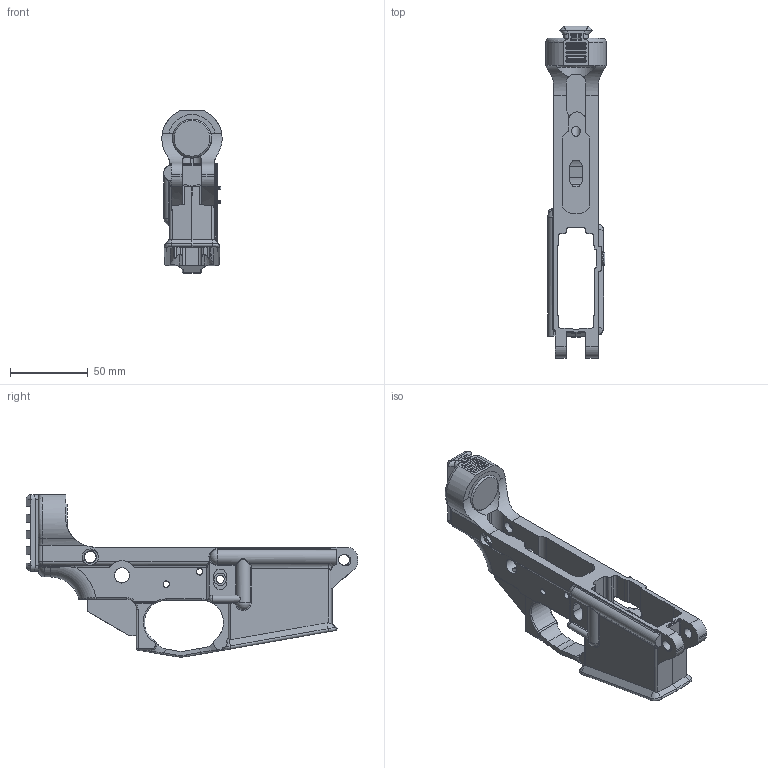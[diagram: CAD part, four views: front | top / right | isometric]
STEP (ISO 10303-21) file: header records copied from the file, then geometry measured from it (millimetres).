
FILE_DESCRIPTION(/* description */ (''),/* implementation_level */ '2;1');
FILE_NAME(/* name */ 'SC1522.step',/* time_stamp */ '2020-10-31T19:11:02-04:00',/* author */ (''),/* organization */ (''),/* preprocessor_version */ 'ST-DEVELOPER v18.1',/* originating_system */ 'Autodesk Translation Framework v9.3.0.1241',/* authorisation */ '');
FILE_SCHEMA (('AUTOMOTIVE_DESIGN { 1 0 10303 214 3 1 1 }'));
Length unit declared in the file: millimetre
Products named in the file (1): SC1522
Bounding box: 38.75 x 213.55 x 104.4 mm (x, y, z)
Volume: 129691 mm3; surface area: 56419.3 mm2
Topology: 2 solids, 2 shells, 555 faces, 1495 edges, 932 vertices
Faces by surface type: cylinder 212, plane 198, bspline 88, torus 37, cone 14, sphere 6
Full cylindrical faces by diameter (mm): 3.962 x2, 4.2 x1, 4.262 x2, 4.9 x1, 5.182 x1, 5.537 x1, 7 x2, 7.475 x2, 7.925 x3, 9.85 x2, 10.476 x2
Entity records: 22540 total; most frequent: CARTESIAN_POINT 9055, ORIENTED_EDGE 2960, DIRECTION 2675, EDGE_CURVE 1480, AXIS2_PLACEMENT_3D 980, VERTEX_POINT 932, LINE 715, VECTOR 715
